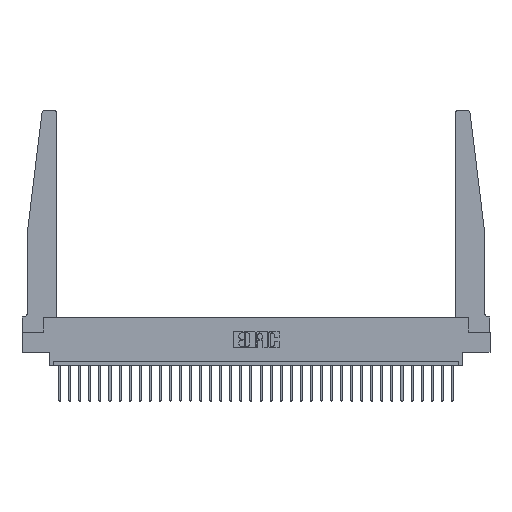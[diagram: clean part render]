
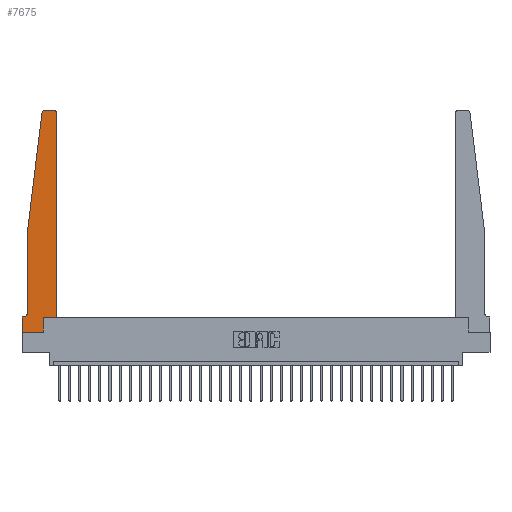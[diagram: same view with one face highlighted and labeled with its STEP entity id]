
A CAD part, top view. The second image highlights one B-rep face of the part: STEP entity #7675.
In plain terms, the highlighted planar face has unit normal (0, 0, 1).
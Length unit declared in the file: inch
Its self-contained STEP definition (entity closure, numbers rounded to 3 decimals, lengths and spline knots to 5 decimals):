
#652 = EDGE_CURVE ( 'NONE', #2600, #27832, #9626, .T. ) ;
#894 = DIRECTION ( 'NONE',  ( 1., 0., 0. ) ) ;
#920 = LINE ( 'NONE', #15305, #22392 ) ;
#1015 = DIRECTION ( 'NONE',  ( -1., 0., 0. ) ) ;
#1101 = VECTOR ( 'NONE', #7295, 39.37008 ) ;
#1180 = AXIS2_PLACEMENT_3D ( 'NONE', #13025, #12584, #15203 ) ;
#1565 = LINE ( 'NONE', #8291, #19675 ) ;
#1633 = CIRCLE ( 'NONE', #8604, 0.05 ) ;
#1797 = ORIENTED_EDGE ( 'NONE', *, *, #15902, .T. ) ;
#2038 = ORIENTED_EDGE ( 'NONE', *, *, #24135, .T. ) ;
#2058 = VERTEX_POINT ( 'NONE', #24481 ) ;
#2370 = VECTOR ( 'NONE', #13838, 39.37008 ) ;
#2383 = DIRECTION ( 'NONE',  ( 0., -1., 0. ) ) ;
#2600 = VERTEX_POINT ( 'NONE', #17872 ) ;
#2768 = EDGE_CURVE ( 'NONE', #6777, #2058, #18473, .T. ) ;
#2779 = VECTOR ( 'NONE', #2383, 39.37008 ) ;
#2840 = CARTESIAN_POINT ( 'NONE',  ( 0.015, 0.2375, 0.37 ) ) ;
#3224 = PLANE ( 'NONE',  #16284 ) ;
#3235 = EDGE_CURVE ( 'NONE', #20071, #22362, #21711, .T. ) ;
#3705 = CARTESIAN_POINT ( 'NONE',  ( 0., 0.1875, 0.37 ) ) ;
#3797 = CARTESIAN_POINT ( 'NONE',  ( 0., 0., 0.37 ) ) ;
#3892 = ORIENTED_EDGE ( 'NONE', *, *, #3235, .T. ) ;
#4346 = DIRECTION ( 'NONE',  ( 0., -1., 0. ) ) ;
#5080 = CARTESIAN_POINT ( 'NONE',  ( 0., 0., 0.37 ) ) ;
#5268 = ORIENTED_EDGE ( 'NONE', *, *, #652, .T. ) ;
#5571 = CARTESIAN_POINT ( 'NONE',  ( 0.24675, 2.72367, 0.37 ) ) ;
#5812 = ORIENTED_EDGE ( 'NONE', *, *, #21471, .T. ) ;
#6054 = ORIENTED_EDGE ( 'NONE', *, *, #12540, .T. ) ;
#6181 = EDGE_CURVE ( 'NONE', #6900, #12481, #1633, .T. ) ;
#6777 = VERTEX_POINT ( 'NONE', #18236 ) ;
#6887 = CARTESIAN_POINT ( 'NONE',  ( 0.065, 1.25, 0.37 ) ) ;
#6900 = VERTEX_POINT ( 'NONE', #20415 ) ;
#7295 = DIRECTION ( 'NONE',  ( 1., 0., 0. ) ) ;
#7528 = CARTESIAN_POINT ( 'NONE',  ( 0.065, 1.25, 0.37 ) ) ;
#7675 = ADVANCED_FACE ( 'NONE', ( #22042 ), #3224, .T. ) ;
#8291 = CARTESIAN_POINT ( 'NONE',  ( 0.425, 0.18, 0.37 ) ) ;
#8604 = AXIS2_PLACEMENT_3D ( 'NONE', #2840, #28264, #23664 ) ;
#8861 = DIRECTION ( 'NONE',  ( 1., 0., 0. ) ) ;
#9248 = CARTESIAN_POINT ( 'NONE',  ( 0.25, 2.75, 0.37 ) ) ;
#9621 = CARTESIAN_POINT ( 'NONE',  ( 0.2605, 0.18, 0.37 ) ) ;
#9626 = LINE ( 'NONE', #28336, #1101 ) ;
#9922 = DIRECTION ( 'NONE',  ( 0., 1., 0. ) ) ;
#10326 = CARTESIAN_POINT ( 'NONE',  ( 0.065, 0.1875, 0.37 ) ) ;
#10369 = EDGE_CURVE ( 'NONE', #23217, #19468, #29184, .T. ) ;
#11907 = ORIENTED_EDGE ( 'NONE', *, *, #24660, .T. ) ;
#12344 = CARTESIAN_POINT ( 'NONE',  ( 0., 0.1875, 0.37 ) ) ;
#12481 = VERTEX_POINT ( 'NONE', #15869 ) ;
#12540 = EDGE_CURVE ( 'NONE', #25601, #20071, #25204, .T. ) ;
#12584 = DIRECTION ( 'NONE',  ( 0., 0., 1. ) ) ;
#12651 = DIRECTION ( 'NONE',  ( 0., 0., 1. ) ) ;
#12966 = VERTEX_POINT ( 'NONE', #6887 ) ;
#13025 = CARTESIAN_POINT ( 'NONE',  ( 0.395, 2.72, 0.37 ) ) ;
#13796 = ORIENTED_EDGE ( 'NONE', *, *, #27777, .T. ) ;
#13838 = DIRECTION ( 'NONE',  ( -1., 0., 0. ) ) ;
#14085 = VECTOR ( 'NONE', #16626, 39.37008 ) ;
#14238 = VECTOR ( 'NONE', #9922, 39.37008 ) ;
#14628 = DIRECTION ( 'NONE',  ( 1., 0., 0. ) ) ;
#15203 = DIRECTION ( 'NONE',  ( 1., 0., 0. ) ) ;
#15248 = LINE ( 'NONE', #9621, #14238 ) ;
#15305 = CARTESIAN_POINT ( 'NONE',  ( 0.065, 1.25, 0.37 ) ) ;
#15869 = CARTESIAN_POINT ( 'NONE',  ( 0.015, 0.1875, 0.37 ) ) ;
#15902 = EDGE_CURVE ( 'NONE', #12481, #25601, #26757, .T. ) ;
#16284 = AXIS2_PLACEMENT_3D ( 'NONE', #12344, #12651, #894 ) ;
#16626 = DIRECTION ( 'NONE',  ( -0.122, -0.992, 0. ) ) ;
#17872 = CARTESIAN_POINT ( 'NONE',  ( 0.2605, 0.18, 0.37 ) ) ;
#18236 = CARTESIAN_POINT ( 'NONE',  ( 0.425, 2.72, 0.37 ) ) ;
#18473 = CIRCLE ( 'NONE', #1180, 0.03 ) ;
#18851 = DIRECTION ( 'NONE',  ( 0., 0., 1. ) ) ;
#19238 = LINE ( 'NONE', #7528, #14085 ) ;
#19391 = ORIENTED_EDGE ( 'NONE', *, *, #10369, .T. ) ;
#19468 = VERTEX_POINT ( 'NONE', #5571 ) ;
#19675 = VECTOR ( 'NONE', #24697, 39.37008 ) ;
#19678 = CARTESIAN_POINT ( 'NONE',  ( 0.27653, 2.75, 0.37 ) ) ;
#20071 = VERTEX_POINT ( 'NONE', #3797 ) ;
#20415 = CARTESIAN_POINT ( 'NONE',  ( 0.065, 0.2375, 0.37 ) ) ;
#20654 = VECTOR ( 'NONE', #1015, 39.37008 ) ;
#21471 = EDGE_CURVE ( 'NONE', #19468, #12966, #19238, .T. ) ;
#21711 = LINE ( 'NONE', #5080, #29540 ) ;
#22042 = FACE_OUTER_BOUND ( 'NONE', #29171, .T. ) ;
#22362 = VERTEX_POINT ( 'NONE', #25881 ) ;
#22392 = VECTOR ( 'NONE', #4346, 39.37008 ) ;
#22571 = ORIENTED_EDGE ( 'NONE', *, *, #6181, .T. ) ;
#22804 = AXIS2_PLACEMENT_3D ( 'NONE', #25732, #18851, #8861 ) ;
#22836 = ORIENTED_EDGE ( 'NONE', *, *, #2768, .T. ) ;
#22955 = CARTESIAN_POINT ( 'NONE',  ( 0.425, 0.18, 0.37 ) ) ;
#23217 = VERTEX_POINT ( 'NONE', #19678 ) ;
#23664 = DIRECTION ( 'NONE',  ( -1., 0., 0. ) ) ;
#24135 = EDGE_CURVE ( 'NONE', #22362, #2600, #15248, .T. ) ;
#24481 = CARTESIAN_POINT ( 'NONE',  ( 0.395, 2.75, 0.37 ) ) ;
#24485 = EDGE_CURVE ( 'NONE', #2058, #23217, #25508, .T. ) ;
#24660 = EDGE_CURVE ( 'NONE', #27832, #6777, #1565, .T. ) ;
#24697 = DIRECTION ( 'NONE',  ( 0., 1., 0. ) ) ;
#25204 = LINE ( 'NONE', #27511, #2779 ) ;
#25508 = LINE ( 'NONE', #9248, #2370 ) ;
#25601 = VERTEX_POINT ( 'NONE', #3705 ) ;
#25732 = CARTESIAN_POINT ( 'NONE',  ( 0.27653, 2.72, 0.37 ) ) ;
#25881 = CARTESIAN_POINT ( 'NONE',  ( 0.2605, 0., 0.37 ) ) ;
#26700 = ORIENTED_EDGE ( 'NONE', *, *, #24485, .T. ) ;
#26757 = LINE ( 'NONE', #10326, #20654 ) ;
#27511 = CARTESIAN_POINT ( 'NONE',  ( 0., 0., 0.37 ) ) ;
#27777 = EDGE_CURVE ( 'NONE', #12966, #6900, #920, .T. ) ;
#27832 = VERTEX_POINT ( 'NONE', #22955 ) ;
#28264 = DIRECTION ( 'NONE',  ( 0., 0., -1. ) ) ;
#28336 = CARTESIAN_POINT ( 'NONE',  ( 0.425, 0.18, 0.37 ) ) ;
#29171 = EDGE_LOOP ( 'NONE', ( #26700, #19391, #5812, #13796, #22571, #1797, #6054, #3892, #2038, #5268, #11907, #22836 ) ) ;
#29184 = CIRCLE ( 'NONE', #22804, 0.03 ) ;
#29540 = VECTOR ( 'NONE', #14628, 39.37008 ) ;
